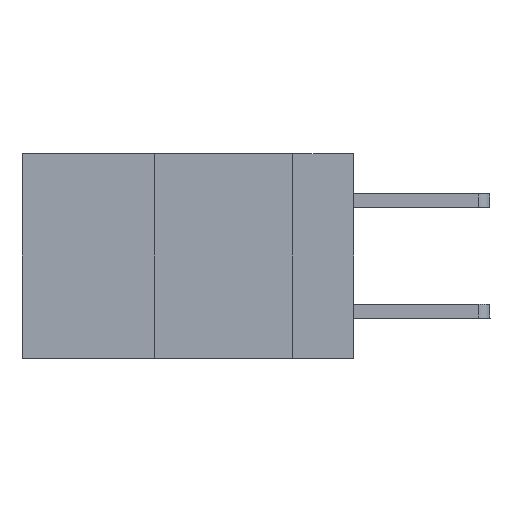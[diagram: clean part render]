
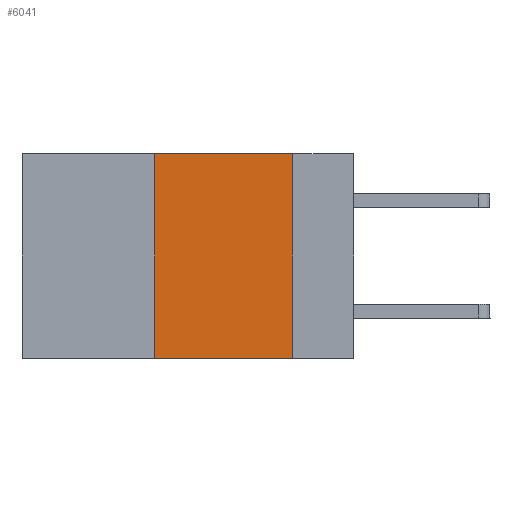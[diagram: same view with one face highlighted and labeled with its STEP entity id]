
A CAD part, left-side view. The second image highlights one B-rep face of the part: STEP entity #6041.
In plain terms, the highlighted planar face has unit normal (-1, 0, 0).
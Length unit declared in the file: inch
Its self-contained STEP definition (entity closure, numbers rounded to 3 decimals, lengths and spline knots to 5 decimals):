
#110 = VERTEX_POINT ( 'NONE', #6142 ) ;
#124 = AXIS2_PLACEMENT_3D ( 'NONE', #6576, #1574, #7729 ) ;
#277 = EDGE_LOOP ( 'NONE', ( #3755, #2731, #9773, #7312 ) ) ;
#465 = FACE_OUTER_BOUND ( 'NONE', #277, .T. ) ;
#1455 = LINE ( 'NONE', #6724, #5593 ) ;
#1574 = DIRECTION ( 'NONE',  ( 1., 0., 0. ) ) ;
#2040 = VERTEX_POINT ( 'NONE', #12380 ) ;
#2731 = ORIENTED_EDGE ( 'NONE', *, *, #7534, .F. ) ;
#3586 = CARTESIAN_POINT ( 'NONE',  ( 0., 0.11, 0. ) ) ;
#3755 = ORIENTED_EDGE ( 'NONE', *, *, #12643, .F. ) ;
#3851 = CARTESIAN_POINT ( 'NONE',  ( 0., 0.6, 0. ) ) ;
#4450 = VERTEX_POINT ( 'NONE', #3586 ) ;
#4601 = DIRECTION ( 'NONE',  ( 0., -1., 0. ) ) ;
#5188 = VECTOR ( 'NONE', #9075, 39.37008 ) ;
#5593 = VECTOR ( 'NONE', #4601, 39.37008 ) ;
#5924 = LINE ( 'NONE', #9015, #5188 ) ;
#6032 = LINE ( 'NONE', #3851, #7156 ) ;
#6041 = ADVANCED_FACE ( 'NONE', ( #465 ), #11845, .F. ) ;
#6142 = CARTESIAN_POINT ( 'NONE',  ( 0., 0.11, -0.37 ) ) ;
#6576 = CARTESIAN_POINT ( 'NONE',  ( 0., 0.6, 0. ) ) ;
#6724 = CARTESIAN_POINT ( 'NONE',  ( 0., 0.6, -0.37 ) ) ;
#6742 = VERTEX_POINT ( 'NONE', #9448 ) ;
#7156 = VECTOR ( 'NONE', #9134, 39.37008 ) ;
#7312 = ORIENTED_EDGE ( 'NONE', *, *, #7406, .T. ) ;
#7406 = EDGE_CURVE ( 'NONE', #6742, #110, #1455, .T. ) ;
#7534 = EDGE_CURVE ( 'NONE', #2040, #4450, #6032, .T. ) ;
#7729 = DIRECTION ( 'NONE',  ( 0., 0., -1. ) ) ;
#8718 = EDGE_CURVE ( 'NONE', #6742, #2040, #5924, .T. ) ;
#9015 = CARTESIAN_POINT ( 'NONE',  ( 0., 0.36, 0. ) ) ;
#9075 = DIRECTION ( 'NONE',  ( 0., 0., 1. ) ) ;
#9122 = VECTOR ( 'NONE', #10303, 39.37008 ) ;
#9134 = DIRECTION ( 'NONE',  ( 0., -1., 0. ) ) ;
#9448 = CARTESIAN_POINT ( 'NONE',  ( 0., 0.36, -0.37 ) ) ;
#9773 = ORIENTED_EDGE ( 'NONE', *, *, #8718, .F. ) ;
#10303 = DIRECTION ( 'NONE',  ( 0., 0., -1. ) ) ;
#11127 = CARTESIAN_POINT ( 'NONE',  ( 0., 0.11, 0. ) ) ;
#11259 = LINE ( 'NONE', #11127, #9122 ) ;
#11845 = PLANE ( 'NONE',  #124 ) ;
#12380 = CARTESIAN_POINT ( 'NONE',  ( 0., 0.36, 0. ) ) ;
#12643 = EDGE_CURVE ( 'NONE', #4450, #110, #11259, .T. ) ;
